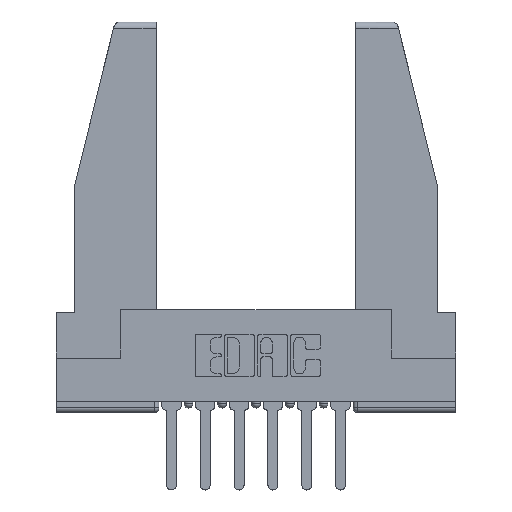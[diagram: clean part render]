
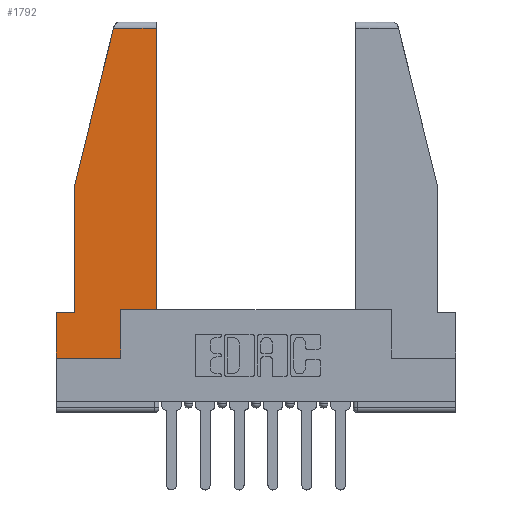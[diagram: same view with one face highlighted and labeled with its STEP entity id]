
A CAD part, top view. The second image highlights one B-rep face of the part: STEP entity #1792.
In plain terms, the highlighted planar face has unit normal (0, 0, 1).
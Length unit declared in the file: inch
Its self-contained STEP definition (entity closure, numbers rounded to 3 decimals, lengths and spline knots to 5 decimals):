
#106 = ORIENTED_EDGE ( 'NONE', *, *, #6268, .T. ) ;
#183 = CARTESIAN_POINT ( 'NONE',  ( 0.271, 1.55, 0. ) ) ;
#342 = ORIENTED_EDGE ( 'NONE', *, *, #11717, .T. ) ;
#381 = DIRECTION ( 'NONE',  ( 0., -1., 0. ) ) ;
#447 = ORIENTED_EDGE ( 'NONE', *, *, #8837, .T. ) ;
#482 = CARTESIAN_POINT ( 'NONE',  ( 0., 0., 0. ) ) ;
#506 = VERTEX_POINT ( 'NONE', #3854 ) ;
#753 = DIRECTION ( 'NONE',  ( 1., 0., 0. ) ) ;
#877 = LINE ( 'NONE', #3233, #8379 ) ;
#1015 = VECTOR ( 'NONE', #10559, 39.37008 ) ;
#1071 = CARTESIAN_POINT ( 'NONE',  ( 0.297, 0., 0. ) ) ;
#1250 = CARTESIAN_POINT ( 'NONE',  ( 0.086, 0.8, 0. ) ) ;
#1509 = ORIENTED_EDGE ( 'NONE', *, *, #8902, .T. ) ;
#1608 = DIRECTION ( 'NONE',  ( 1., 0., 0. ) ) ;
#1615 = CARTESIAN_POINT ( 'NONE',  ( 0., 1.52, 0. ) ) ;
#1651 = FACE_OUTER_BOUND ( 'NONE', #2219, .T. ) ;
#1740 = LINE ( 'NONE', #1615, #8780 ) ;
#1785 = DIRECTION ( 'NONE',  ( -1., 0., 0. ) ) ;
#1792 = ADVANCED_FACE ( 'NONE', ( #1651 ), #12037, .T. ) ;
#2219 = EDGE_LOOP ( 'NONE', ( #3344, #3411, #447, #1509, #12125, #10661, #106, #8157, #342 ) ) ;
#2476 = VERTEX_POINT ( 'NONE', #9435 ) ;
#2800 = DIRECTION ( 'NONE',  ( -1., 0., 0. ) ) ;
#3233 = CARTESIAN_POINT ( 'NONE',  ( 0.297, 0.223, 0. ) ) ;
#3283 = CARTESIAN_POINT ( 'NONE',  ( 0.086, 0.8, 0. ) ) ;
#3344 = ORIENTED_EDGE ( 'NONE', *, *, #7786, .T. ) ;
#3411 = ORIENTED_EDGE ( 'NONE', *, *, #3887, .T. ) ;
#3762 = VECTOR ( 'NONE', #11953, 39.37008 ) ;
#3778 = VERTEX_POINT ( 'NONE', #482 ) ;
#3848 = LINE ( 'NONE', #8396, #5622 ) ;
#3854 = CARTESIAN_POINT ( 'NONE',  ( 0.086, 0.21, 0. ) ) ;
#3887 = EDGE_CURVE ( 'NONE', #2476, #10931, #1740, .T. ) ;
#4007 = VECTOR ( 'NONE', #1608, 39.37008 ) ;
#4242 = CARTESIAN_POINT ( 'NONE',  ( 0.461, 0.223, 0. ) ) ;
#4362 = VERTEX_POINT ( 'NONE', #4242 ) ;
#5622 = VECTOR ( 'NONE', #2800, 39.37008 ) ;
#5709 = CARTESIAN_POINT ( 'NONE',  ( 0.297, 0., 0. ) ) ;
#6066 = DIRECTION ( 'NONE',  ( 1., 0., 0. ) ) ;
#6162 = CARTESIAN_POINT ( 'NONE',  ( 0.297, 0.223, 0. ) ) ;
#6268 = EDGE_CURVE ( 'NONE', #3778, #11390, #10638, .T. ) ;
#6384 = EDGE_CURVE ( 'NONE', #506, #12062, #3848, .T. ) ;
#6407 = CARTESIAN_POINT ( 'NONE',  ( 0.2636, 1.52, 0. ) ) ;
#6692 = LINE ( 'NONE', #1071, #8020 ) ;
#7409 = DIRECTION ( 'NONE',  ( 0., 0., 1. ) ) ;
#7596 = VECTOR ( 'NONE', #10628, 39.37008 ) ;
#7786 = EDGE_CURVE ( 'NONE', #4362, #2476, #8968, .T. ) ;
#7788 = CARTESIAN_POINT ( 'NONE',  ( 0.461, 0.223, 0. ) ) ;
#8020 = VECTOR ( 'NONE', #8875, 39.37008 ) ;
#8157 = ORIENTED_EDGE ( 'NONE', *, *, #10621, .T. ) ;
#8379 = VECTOR ( 'NONE', #6066, 39.37008 ) ;
#8396 = CARTESIAN_POINT ( 'NONE',  ( 0., 0.21, 0. ) ) ;
#8595 = LINE ( 'NONE', #9265, #3762 ) ;
#8780 = VECTOR ( 'NONE', #1785, 39.37008 ) ;
#8786 = LINE ( 'NONE', #3283, #11013 ) ;
#8837 = EDGE_CURVE ( 'NONE', #10931, #11471, #9086, .T. ) ;
#8875 = DIRECTION ( 'NONE',  ( 0., 1., 0. ) ) ;
#8902 = EDGE_CURVE ( 'NONE', #11471, #506, #8786, .T. ) ;
#8968 = LINE ( 'NONE', #7788, #1015 ) ;
#9086 = LINE ( 'NONE', #183, #7596 ) ;
#9102 = CARTESIAN_POINT ( 'NONE',  ( 0., 0., 0. ) ) ;
#9265 = CARTESIAN_POINT ( 'NONE',  ( 0., 0.21, 0. ) ) ;
#9435 = CARTESIAN_POINT ( 'NONE',  ( 0.461, 1.52, 0. ) ) ;
#9978 = AXIS2_PLACEMENT_3D ( 'NONE', #10304, #7409, #753 ) ;
#10223 = EDGE_CURVE ( 'NONE', #12062, #3778, #8595, .T. ) ;
#10304 = CARTESIAN_POINT ( 'NONE',  ( 0., 0., 0. ) ) ;
#10559 = DIRECTION ( 'NONE',  ( 0., 1., 0. ) ) ;
#10621 = EDGE_CURVE ( 'NONE', #11390, #10827, #6692, .T. ) ;
#10628 = DIRECTION ( 'NONE',  ( -0.239, -0.971, 0. ) ) ;
#10638 = LINE ( 'NONE', #9102, #4007 ) ;
#10661 = ORIENTED_EDGE ( 'NONE', *, *, #10223, .T. ) ;
#10827 = VERTEX_POINT ( 'NONE', #6162 ) ;
#10931 = VERTEX_POINT ( 'NONE', #6407 ) ;
#11013 = VECTOR ( 'NONE', #381, 39.37008 ) ;
#11390 = VERTEX_POINT ( 'NONE', #5709 ) ;
#11471 = VERTEX_POINT ( 'NONE', #1250 ) ;
#11717 = EDGE_CURVE ( 'NONE', #10827, #4362, #877, .T. ) ;
#11953 = DIRECTION ( 'NONE',  ( 0., -1., 0. ) ) ;
#12037 = PLANE ( 'NONE',  #9978 ) ;
#12062 = VERTEX_POINT ( 'NONE', #12096 ) ;
#12096 = CARTESIAN_POINT ( 'NONE',  ( 0., 0.21, 0. ) ) ;
#12125 = ORIENTED_EDGE ( 'NONE', *, *, #6384, .T. ) ;
